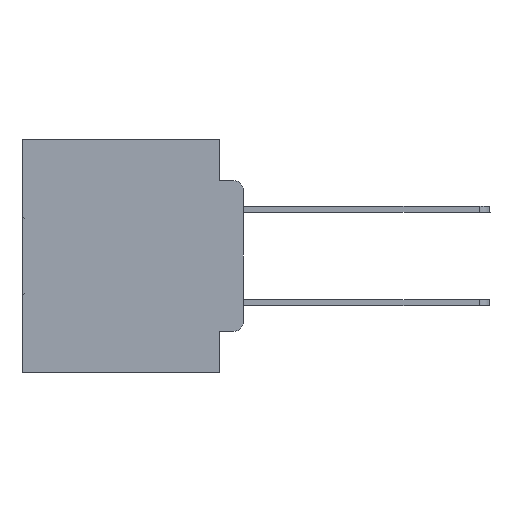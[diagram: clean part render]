
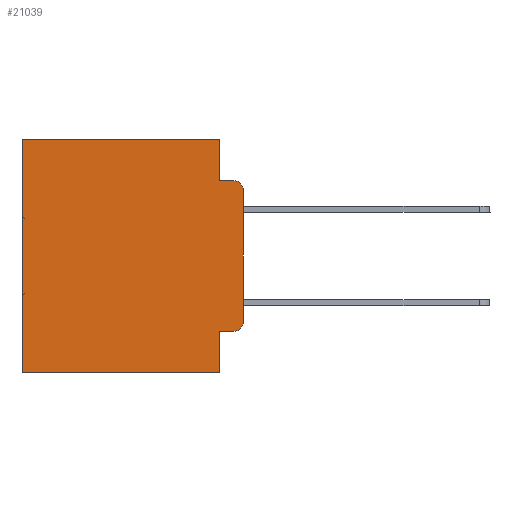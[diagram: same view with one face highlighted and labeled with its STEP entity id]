
A CAD part, left-side view. The second image highlights one B-rep face of the part: STEP entity #21039.
In plain terms, the highlighted planar face has unit normal (-1, 0, 0).
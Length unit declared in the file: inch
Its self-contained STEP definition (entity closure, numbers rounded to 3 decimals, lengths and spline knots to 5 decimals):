
#414 = VECTOR ( 'NONE', #4384, 39.37008 ) ;
#1213 = CARTESIAN_POINT ( 'NONE',  ( 0.298, 0., 0. ) ) ;
#1411 = VECTOR ( 'NONE', #20555, 39.37008 ) ;
#1798 = CARTESIAN_POINT ( 'NONE',  ( 0.298, 0.473, 0. ) ) ;
#2196 = EDGE_CURVE ( 'NONE', #15413, #2653, #6787, .T. ) ;
#2632 = CARTESIAN_POINT ( 'NONE',  ( 0.298, 0., 0. ) ) ;
#2653 = VERTEX_POINT ( 'NONE', #31139 ) ;
#3006 = CARTESIAN_POINT ( 'NONE',  ( 0.298, 0., -0.1085 ) ) ;
#3612 = ORIENTED_EDGE ( 'NONE', *, *, #25192, .T. ) ;
#3688 = DIRECTION ( 'NONE',  ( 0., -1., 0. ) ) ;
#3725 = VERTEX_POINT ( 'NONE', #8708 ) ;
#3798 = FACE_OUTER_BOUND ( 'NONE', #11799, .T. ) ;
#3970 = DIRECTION ( 'NONE',  ( -1., 0., 0. ) ) ;
#4384 = DIRECTION ( 'NONE',  ( 0., 0., -1. ) ) ;
#4469 = DIRECTION ( 'NONE',  ( 0., 0., -1. ) ) ;
#4516 = CARTESIAN_POINT ( 'NONE',  ( 0.298, 0.051, 0. ) ) ;
#4604 = VECTOR ( 'NONE', #3688, 39.37008 ) ;
#4771 = CARTESIAN_POINT ( 'NONE',  ( 0.298, 0., -0.5 ) ) ;
#4873 = CARTESIAN_POINT ( 'NONE',  ( 0.298, 0.02, -0.0885 ) ) ;
#5106 = AXIS2_PLACEMENT_3D ( 'NONE', #1213, #14798, #4469 ) ;
#5222 = ORIENTED_EDGE ( 'NONE', *, *, #26735, .T. ) ;
#5228 = ORIENTED_EDGE ( 'NONE', *, *, #8872, .T. ) ;
#5459 = CARTESIAN_POINT ( 'NONE',  ( 0.298, 0.051, -0.4115 ) ) ;
#6077 = DIRECTION ( 'NONE',  ( 0., 0., -1. ) ) ;
#6295 = LINE ( 'NONE', #9054, #4604 ) ;
#6787 = LINE ( 'NONE', #4516, #7882 ) ;
#7078 = PLANE ( 'NONE',  #5106 ) ;
#7686 = ORIENTED_EDGE ( 'NONE', *, *, #27889, .T. ) ;
#7882 = VECTOR ( 'NONE', #17281, 39.37008 ) ;
#8344 = DIRECTION ( 'NONE',  ( -1., 0., 0. ) ) ;
#8377 = AXIS2_PLACEMENT_3D ( 'NONE', #8514, #8344, #18846 ) ;
#8514 = CARTESIAN_POINT ( 'NONE',  ( 0.298, 0.02, -0.3915 ) ) ;
#8631 = ORIENTED_EDGE ( 'NONE', *, *, #12561, .F. ) ;
#8678 = ORIENTED_EDGE ( 'NONE', *, *, #27798, .F. ) ;
#8708 = CARTESIAN_POINT ( 'NONE',  ( 0.298, 0.473, -0.5 ) ) ;
#8818 = VERTEX_POINT ( 'NONE', #19015 ) ;
#8872 = EDGE_CURVE ( 'NONE', #22513, #24509, #31405, .T. ) ;
#9054 = CARTESIAN_POINT ( 'NONE',  ( 0.298, 0.051, -0.0885 ) ) ;
#9874 = VERTEX_POINT ( 'NONE', #18992 ) ;
#11659 = DIRECTION ( 'NONE',  ( 0., 0., -1. ) ) ;
#11799 = EDGE_LOOP ( 'NONE', ( #13206, #5222, #8631, #8678, #28471, #7686, #15716, #12110, #3612, #5228 ) ) ;
#12110 = ORIENTED_EDGE ( 'NONE', *, *, #2196, .F. ) ;
#12561 = EDGE_CURVE ( 'NONE', #9874, #24536, #6295, .T. ) ;
#12973 = LINE ( 'NONE', #2632, #1411 ) ;
#13206 = ORIENTED_EDGE ( 'NONE', *, *, #14562, .F. ) ;
#14562 = EDGE_CURVE ( 'NONE', #24129, #24509, #12973, .T. ) ;
#14668 = CARTESIAN_POINT ( 'NONE',  ( 0.298, 0.051, 0. ) ) ;
#14798 = DIRECTION ( 'NONE',  ( 1., 0., 0. ) ) ;
#15413 = VERTEX_POINT ( 'NONE', #5459 ) ;
#15716 = ORIENTED_EDGE ( 'NONE', *, *, #30720, .F. ) ;
#16297 = CARTESIAN_POINT ( 'NONE',  ( 0.298, 0.02, -0.4115 ) ) ;
#17281 = DIRECTION ( 'NONE',  ( 0., 0., -1. ) ) ;
#17354 = LINE ( 'NONE', #4771, #27437 ) ;
#17959 = CARTESIAN_POINT ( 'NONE',  ( 0.298, 0., -0.3915 ) ) ;
#18069 = VECTOR ( 'NONE', #26836, 39.37008 ) ;
#18846 = DIRECTION ( 'NONE',  ( 0., 0., -1. ) ) ;
#18992 = CARTESIAN_POINT ( 'NONE',  ( 0.298, 0.051, -0.0885 ) ) ;
#19015 = CARTESIAN_POINT ( 'NONE',  ( 0.298, 0.473, 0. ) ) ;
#19412 = VERTEX_POINT ( 'NONE', #14668 ) ;
#20555 = DIRECTION ( 'NONE',  ( 0., 0., -1. ) ) ;
#20678 = AXIS2_PLACEMENT_3D ( 'NONE', #27570, #3970, #6077 ) ;
#21039 = ADVANCED_FACE ( 'NONE', ( #3798 ), #7078, .F. ) ;
#21989 = LINE ( 'NONE', #32466, #31600 ) ;
#22154 = DIRECTION ( 'NONE',  ( 0., -1., 0. ) ) ;
#22513 = VERTEX_POINT ( 'NONE', #16297 ) ;
#24129 = VERTEX_POINT ( 'NONE', #3006 ) ;
#24509 = VERTEX_POINT ( 'NONE', #17959 ) ;
#24536 = VERTEX_POINT ( 'NONE', #4873 ) ;
#25192 = EDGE_CURVE ( 'NONE', #15413, #22513, #21989, .T. ) ;
#25237 = CARTESIAN_POINT ( 'NONE',  ( 0.298, 0.051, 0. ) ) ;
#25771 = DIRECTION ( 'NONE',  ( 0., 1., 0. ) ) ;
#26735 = EDGE_CURVE ( 'NONE', #24129, #24536, #26739, .T. ) ;
#26739 = CIRCLE ( 'NONE', #20678, 0.02 ) ;
#26836 = DIRECTION ( 'NONE',  ( 0., 1., 0. ) ) ;
#27006 = CARTESIAN_POINT ( 'NONE',  ( 0.298, 0., 0. ) ) ;
#27437 = VECTOR ( 'NONE', #25771, 39.37008 ) ;
#27570 = CARTESIAN_POINT ( 'NONE',  ( 0.298, 0.02, -0.1085 ) ) ;
#27798 = EDGE_CURVE ( 'NONE', #19412, #9874, #30373, .T. ) ;
#27889 = EDGE_CURVE ( 'NONE', #8818, #3725, #30207, .T. ) ;
#28471 = ORIENTED_EDGE ( 'NONE', *, *, #29031, .T. ) ;
#29031 = EDGE_CURVE ( 'NONE', #19412, #8818, #29897, .T. ) ;
#29538 = VECTOR ( 'NONE', #11659, 39.37008 ) ;
#29897 = LINE ( 'NONE', #27006, #18069 ) ;
#30207 = LINE ( 'NONE', #1798, #414 ) ;
#30373 = LINE ( 'NONE', #25237, #29538 ) ;
#30720 = EDGE_CURVE ( 'NONE', #2653, #3725, #17354, .T. ) ;
#31139 = CARTESIAN_POINT ( 'NONE',  ( 0.298, 0.051, -0.5 ) ) ;
#31405 = CIRCLE ( 'NONE', #8377, 0.02 ) ;
#31600 = VECTOR ( 'NONE', #22154, 39.37008 ) ;
#32466 = CARTESIAN_POINT ( 'NONE',  ( 0.298, 0.051, -0.4115 ) ) ;
